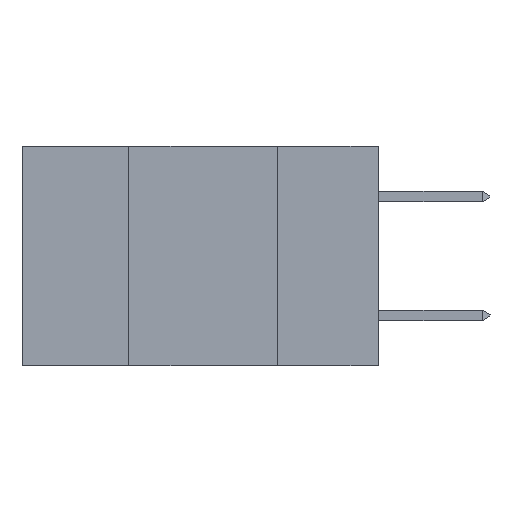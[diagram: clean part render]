
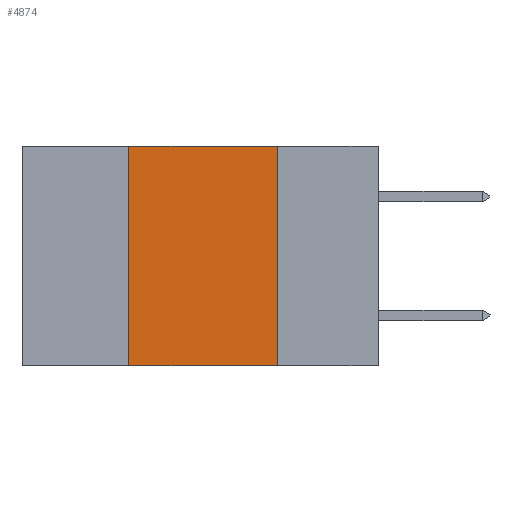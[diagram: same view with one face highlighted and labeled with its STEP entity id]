
A CAD part, left-side view. The second image highlights one B-rep face of the part: STEP entity #4874.
In plain terms, the highlighted planar face has unit normal (-1, 0, 0).
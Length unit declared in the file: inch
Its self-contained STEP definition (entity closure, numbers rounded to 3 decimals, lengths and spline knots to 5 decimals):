
#855 = PLANE ( 'NONE',  #10173 ) ;
#987 = VECTOR ( 'NONE', #9429, 39.37008 ) ;
#1074 = CARTESIAN_POINT ( 'NONE',  ( 0., 0.6, -0.37 ) ) ;
#1375 = VECTOR ( 'NONE', #7544, 39.37008 ) ;
#1885 = DIRECTION ( 'NONE',  ( 0., 0., -1. ) ) ;
#2163 = EDGE_CURVE ( 'NONE', #9050, #2955, #8470, .T. ) ;
#2429 = VECTOR ( 'NONE', #12809, 39.37008 ) ;
#2822 = LINE ( 'NONE', #1074, #987 ) ;
#2839 = CARTESIAN_POINT ( 'NONE',  ( 0., 0.6, 0. ) ) ;
#2955 = VERTEX_POINT ( 'NONE', #11085 ) ;
#4041 = EDGE_LOOP ( 'NONE', ( #6910, #11017, #7535, #8076 ) ) ;
#4315 = FACE_OUTER_BOUND ( 'NONE', #4041, .T. ) ;
#4416 = CARTESIAN_POINT ( 'NONE',  ( 0., 0.17, 0. ) ) ;
#4568 = EDGE_CURVE ( 'NONE', #7145, #11108, #2822, .T. ) ;
#4627 = CARTESIAN_POINT ( 'NONE',  ( 0., 0.42, 0. ) ) ;
#4654 = VECTOR ( 'NONE', #11917, 39.37008 ) ;
#4874 = ADVANCED_FACE ( 'NONE', ( #4315 ), #855, .F. ) ;
#5612 = LINE ( 'NONE', #10917, #4654 ) ;
#6910 = ORIENTED_EDGE ( 'NONE', *, *, #13764, .F. ) ;
#7145 = VERTEX_POINT ( 'NONE', #11662 ) ;
#7535 = ORIENTED_EDGE ( 'NONE', *, *, #14514, .F. ) ;
#7544 = DIRECTION ( 'NONE',  ( 0., -1., 0. ) ) ;
#7863 = CARTESIAN_POINT ( 'NONE',  ( 0., 0.17, -0.37 ) ) ;
#8076 = ORIENTED_EDGE ( 'NONE', *, *, #4568, .T. ) ;
#8470 = LINE ( 'NONE', #2839, #1375 ) ;
#9050 = VERTEX_POINT ( 'NONE', #4627 ) ;
#9200 = CARTESIAN_POINT ( 'NONE',  ( 0., 0.6, 0. ) ) ;
#9429 = DIRECTION ( 'NONE',  ( 0., -1., 0. ) ) ;
#10173 = AXIS2_PLACEMENT_3D ( 'NONE', #9200, #12325, #1885 ) ;
#10917 = CARTESIAN_POINT ( 'NONE',  ( 0., 0.42, 0. ) ) ;
#11017 = ORIENTED_EDGE ( 'NONE', *, *, #2163, .F. ) ;
#11036 = LINE ( 'NONE', #4416, #2429 ) ;
#11085 = CARTESIAN_POINT ( 'NONE',  ( 0., 0.17, 0. ) ) ;
#11108 = VERTEX_POINT ( 'NONE', #7863 ) ;
#11662 = CARTESIAN_POINT ( 'NONE',  ( 0., 0.42, -0.37 ) ) ;
#11917 = DIRECTION ( 'NONE',  ( 0., 0., 1. ) ) ;
#12325 = DIRECTION ( 'NONE',  ( 1., 0., 0. ) ) ;
#12809 = DIRECTION ( 'NONE',  ( 0., 0., -1. ) ) ;
#13764 = EDGE_CURVE ( 'NONE', #2955, #11108, #11036, .T. ) ;
#14514 = EDGE_CURVE ( 'NONE', #7145, #9050, #5612, .T. ) ;
